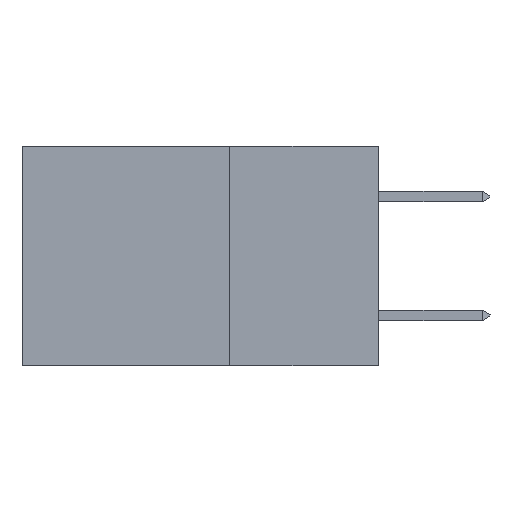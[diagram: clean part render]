
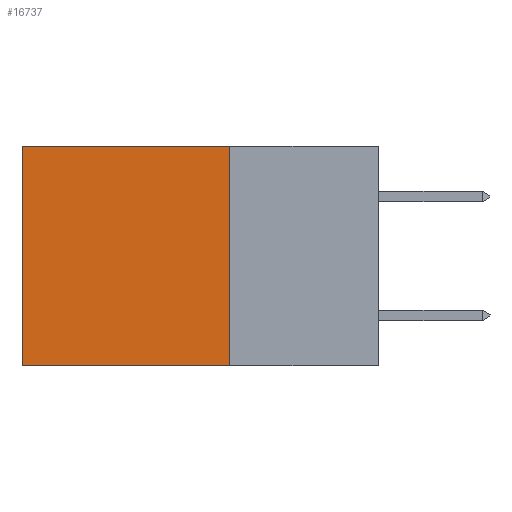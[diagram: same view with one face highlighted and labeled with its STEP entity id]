
A CAD part, left-side view. The second image highlights one B-rep face of the part: STEP entity #16737.
In plain terms, the highlighted planar face has unit normal (-1, 0, 0).
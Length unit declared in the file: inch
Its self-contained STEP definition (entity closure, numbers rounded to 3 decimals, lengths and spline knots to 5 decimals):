
#1484 = VERTEX_POINT ( 'NONE', #21479 ) ;
#1876 = CARTESIAN_POINT ( 'NONE',  ( 0.298, 0.6, 0. ) ) ;
#2538 = DIRECTION ( 'NONE',  ( 1., 0., 0. ) ) ;
#3387 = CARTESIAN_POINT ( 'NONE',  ( 0.298, 0.25, 0. ) ) ;
#3892 = EDGE_CURVE ( 'NONE', #1484, #13535, #22123, .T. ) ;
#4167 = VERTEX_POINT ( 'NONE', #17814 ) ;
#4821 = CARTESIAN_POINT ( 'NONE',  ( 0.298, 0.25, -0.37 ) ) ;
#5134 = ORIENTED_EDGE ( 'NONE', *, *, #14179, .T. ) ;
#5595 = LINE ( 'NONE', #16107, #10122 ) ;
#6949 = LINE ( 'NONE', #3387, #23631 ) ;
#7367 = ORIENTED_EDGE ( 'NONE', *, *, #3892, .F. ) ;
#8671 = EDGE_LOOP ( 'NONE', ( #22811, #7367, #15249, #5134 ) ) ;
#10122 = VECTOR ( 'NONE', #16630, 39.37008 ) ;
#10180 = FACE_OUTER_BOUND ( 'NONE', #8671, .T. ) ;
#10707 = EDGE_CURVE ( 'NONE', #14995, #13535, #16352, .T. ) ;
#11462 = DIRECTION ( 'NONE',  ( 0., 1., 0. ) ) ;
#12151 = PLANE ( 'NONE',  #22738 ) ;
#13535 = VERTEX_POINT ( 'NONE', #15908 ) ;
#14179 = EDGE_CURVE ( 'NONE', #4167, #14995, #6949, .T. ) ;
#14995 = VERTEX_POINT ( 'NONE', #25594 ) ;
#15249 = ORIENTED_EDGE ( 'NONE', *, *, #15645, .F. ) ;
#15645 = EDGE_CURVE ( 'NONE', #4167, #1484, #5595, .T. ) ;
#15892 = VECTOR ( 'NONE', #24434, 39.37008 ) ;
#15908 = CARTESIAN_POINT ( 'NONE',  ( 0.298, 0.6, -0.37 ) ) ;
#16107 = CARTESIAN_POINT ( 'NONE',  ( 0.298, 0.25, 0. ) ) ;
#16290 = DIRECTION ( 'NONE',  ( 0., 0., -1. ) ) ;
#16352 = LINE ( 'NONE', #1876, #20696 ) ;
#16630 = DIRECTION ( 'NONE',  ( 0., 0., -1. ) ) ;
#16737 = ADVANCED_FACE ( 'NONE', ( #10180 ), #12151, .F. ) ;
#17616 = DIRECTION ( 'NONE',  ( 0., 0., -1. ) ) ;
#17814 = CARTESIAN_POINT ( 'NONE',  ( 0.298, 0.25, 0. ) ) ;
#20186 = CARTESIAN_POINT ( 'NONE',  ( 0.298, 0.25, 0. ) ) ;
#20696 = VECTOR ( 'NONE', #17616, 39.37008 ) ;
#21479 = CARTESIAN_POINT ( 'NONE',  ( 0.298, 0.25, -0.37 ) ) ;
#22123 = LINE ( 'NONE', #4821, #15892 ) ;
#22738 = AXIS2_PLACEMENT_3D ( 'NONE', #20186, #2538, #16290 ) ;
#22811 = ORIENTED_EDGE ( 'NONE', *, *, #10707, .T. ) ;
#23631 = VECTOR ( 'NONE', #11462, 39.37008 ) ;
#24434 = DIRECTION ( 'NONE',  ( 0., 1., 0. ) ) ;
#25594 = CARTESIAN_POINT ( 'NONE',  ( 0.298, 0.6, 0. ) ) ;
